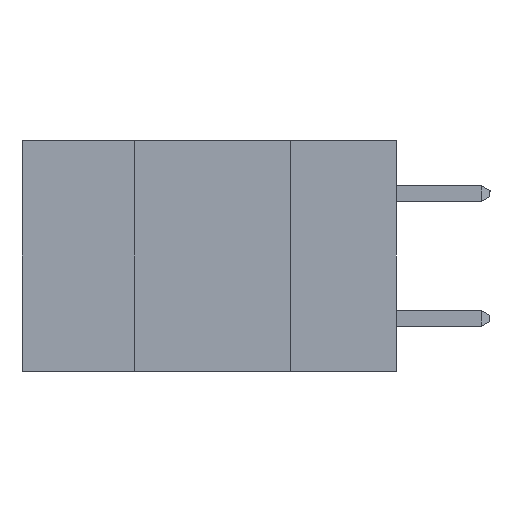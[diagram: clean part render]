
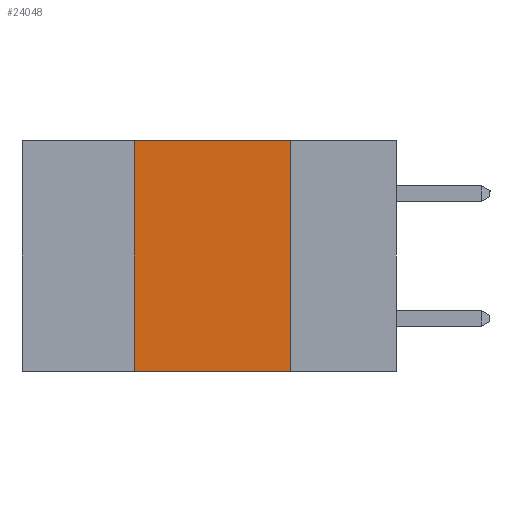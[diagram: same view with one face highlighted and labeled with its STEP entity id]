
A CAD part, left-side view. The second image highlights one B-rep face of the part: STEP entity #24048.
In plain terms, the highlighted planar face has unit normal (-1, 0, 0).
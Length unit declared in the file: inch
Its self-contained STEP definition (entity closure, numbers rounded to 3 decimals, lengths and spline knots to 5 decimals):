
#1058 = EDGE_CURVE ( 'NONE', #13449, #20759, #8946, .T. ) ;
#2121 = FACE_OUTER_BOUND ( 'NONE', #14023, .T. ) ;
#2280 = ORIENTED_EDGE ( 'NONE', *, *, #7702, .F. ) ;
#2658 = VECTOR ( 'NONE', #17222, 39.37008 ) ;
#3826 = CARTESIAN_POINT ( 'NONE',  ( 0., 0.42, -0.37 ) ) ;
#4809 = VECTOR ( 'NONE', #13309, 39.37008 ) ;
#7528 = CARTESIAN_POINT ( 'NONE',  ( 0., 0.17, -0.37 ) ) ;
#7663 = DIRECTION ( 'NONE',  ( 0., 0., -1. ) ) ;
#7683 = LINE ( 'NONE', #3826, #4809 ) ;
#7702 = EDGE_CURVE ( 'NONE', #13449, #17935, #7683, .T. ) ;
#8550 = DIRECTION ( 'NONE',  ( 0., -1., 0. ) ) ;
#8798 = CARTESIAN_POINT ( 'NONE',  ( 0., 0.6, 0. ) ) ;
#8946 = LINE ( 'NONE', #16840, #10722 ) ;
#9192 = DIRECTION ( 'NONE',  ( 0., -1., 0. ) ) ;
#9849 = PLANE ( 'NONE',  #14185 ) ;
#10722 = VECTOR ( 'NONE', #9192, 39.37008 ) ;
#11439 = CARTESIAN_POINT ( 'NONE',  ( 0., 0.17, -0.37 ) ) ;
#11843 = ORIENTED_EDGE ( 'NONE', *, *, #12121, .F. ) ;
#11916 = EDGE_CURVE ( 'NONE', #17935, #18162, #14668, .T. ) ;
#12121 = EDGE_CURVE ( 'NONE', #18162, #20759, #24649, .T. ) ;
#12515 = ORIENTED_EDGE ( 'NONE', *, *, #1058, .T. ) ;
#13309 = DIRECTION ( 'NONE',  ( 0., 0., 1. ) ) ;
#13434 = CARTESIAN_POINT ( 'NONE',  ( 0., 0.42, 0. ) ) ;
#13449 = VERTEX_POINT ( 'NONE', #21629 ) ;
#14023 = EDGE_LOOP ( 'NONE', ( #11843, #20355, #2280, #12515 ) ) ;
#14185 = AXIS2_PLACEMENT_3D ( 'NONE', #19405, #17356, #7663 ) ;
#14290 = CARTESIAN_POINT ( 'NONE',  ( 0., 0.17, 0. ) ) ;
#14668 = LINE ( 'NONE', #8798, #17554 ) ;
#16840 = CARTESIAN_POINT ( 'NONE',  ( 0., 0.6, -0.37 ) ) ;
#17222 = DIRECTION ( 'NONE',  ( 0., 0., -1. ) ) ;
#17356 = DIRECTION ( 'NONE',  ( 1., 0., 0. ) ) ;
#17554 = VECTOR ( 'NONE', #8550, 39.37008 ) ;
#17935 = VERTEX_POINT ( 'NONE', #13434 ) ;
#18162 = VERTEX_POINT ( 'NONE', #14290 ) ;
#19405 = CARTESIAN_POINT ( 'NONE',  ( 0., 0.6, 0. ) ) ;
#20355 = ORIENTED_EDGE ( 'NONE', *, *, #11916, .F. ) ;
#20759 = VERTEX_POINT ( 'NONE', #11439 ) ;
#21629 = CARTESIAN_POINT ( 'NONE',  ( 0., 0.42, -0.37 ) ) ;
#24048 = ADVANCED_FACE ( 'NONE', ( #2121 ), #9849, .F. ) ;
#24649 = LINE ( 'NONE', #7528, #2658 ) ;
